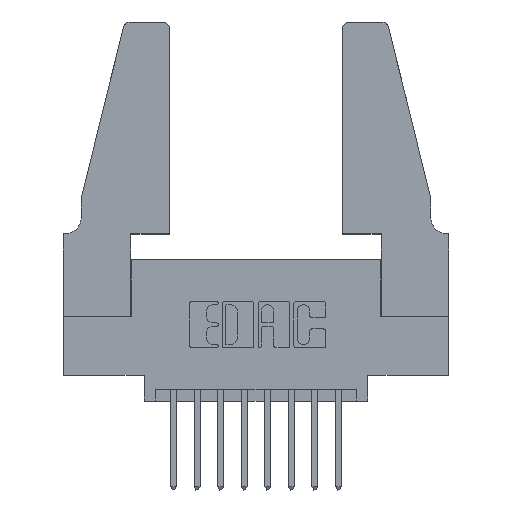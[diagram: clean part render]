
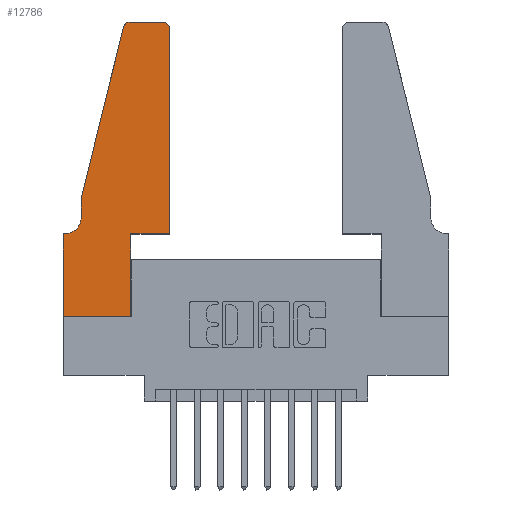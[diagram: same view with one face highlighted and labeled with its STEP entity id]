
A CAD part, top view. The second image highlights one B-rep face of the part: STEP entity #12786.
In plain terms, the highlighted planar face has unit normal (0, 0, 1).
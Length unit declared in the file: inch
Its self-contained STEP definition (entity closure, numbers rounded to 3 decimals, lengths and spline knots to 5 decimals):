
#7 = DIRECTION ( 'NONE',  ( 0., 1., 0. ) ) ;
#111 = CARTESIAN_POINT ( 'NONE',  ( 0.284, 1.22, 0.37 ) ) ;
#139 = VECTOR ( 'NONE', #7, 39.37008 ) ;
#411 = VERTEX_POINT ( 'NONE', #1098 ) ;
#494 = LINE ( 'NONE', #7327, #139 ) ;
#654 = ORIENTED_EDGE ( 'NONE', *, *, #11352, .T. ) ;
#858 = LINE ( 'NONE', #7515, #8776 ) ;
#988 = DIRECTION ( 'NONE',  ( -1., 0., 0. ) ) ;
#1098 = CARTESIAN_POINT ( 'NONE',  ( 0.284, 1.25, 0.37 ) ) ;
#1178 = VECTOR ( 'NONE', #6517, 39.37008 ) ;
#1212 = DIRECTION ( 'NONE',  ( 1., 0., 0. ) ) ;
#1305 = DIRECTION ( 'NONE',  ( 0., -1., 0. ) ) ;
#1390 = ORIENTED_EDGE ( 'NONE', *, *, #6746, .T. ) ;
#1464 = CARTESIAN_POINT ( 'NONE',  ( 0.4505, 0.35, 0.37 ) ) ;
#1557 = ORIENTED_EDGE ( 'NONE', *, *, #8602, .T. ) ;
#1567 = CARTESIAN_POINT ( 'NONE',  ( 0.0055, 0.42, 0.37 ) ) ;
#1568 = EDGE_LOOP ( 'NONE', ( #2621, #1390, #12652, #9946, #3167, #3670, #12107, #654, #2486, #9514, #1557, #12460 ) ) ;
#2068 = CARTESIAN_POINT ( 'NONE',  ( 0.0755, 0.35, 0.37 ) ) ;
#2070 = AXIS2_PLACEMENT_3D ( 'NONE', #9506, #10512, #4467 ) ;
#2393 = PLANE ( 'NONE',  #2070 ) ;
#2395 = LINE ( 'NONE', #2068, #12779 ) ;
#2486 = ORIENTED_EDGE ( 'NONE', *, *, #5365, .T. ) ;
#2611 = CARTESIAN_POINT ( 'NONE',  ( 0.2865, 0.35, 0.37 ) ) ;
#2621 = ORIENTED_EDGE ( 'NONE', *, *, #4824, .T. ) ;
#2660 = DIRECTION ( 'NONE',  ( -1., 0., 0. ) ) ;
#2668 = VECTOR ( 'NONE', #8223, 39.37008 ) ;
#3029 = LINE ( 'NONE', #4763, #10786 ) ;
#3167 = ORIENTED_EDGE ( 'NONE', *, *, #9103, .T. ) ;
#3335 = VECTOR ( 'NONE', #6585, 39.37008 ) ;
#3392 = VERTEX_POINT ( 'NONE', #5178 ) ;
#3670 = ORIENTED_EDGE ( 'NONE', *, *, #4068, .T. ) ;
#3869 = DIRECTION ( 'NONE',  ( 0., 0., 1. ) ) ;
#4068 = EDGE_CURVE ( 'NONE', #4286, #9847, #2395, .T. ) ;
#4286 = VERTEX_POINT ( 'NONE', #10531 ) ;
#4381 = AXIS2_PLACEMENT_3D ( 'NONE', #111, #7429, #1212 ) ;
#4429 = CARTESIAN_POINT ( 'NONE',  ( 0.2605, 1.25, 0.37 ) ) ;
#4467 = DIRECTION ( 'NONE',  ( 1., 0., 0. ) ) ;
#4750 = EDGE_CURVE ( 'NONE', #7225, #6259, #4949, .T. ) ;
#4763 = CARTESIAN_POINT ( 'NONE',  ( 0.4505, 0.35, 0.37 ) ) ;
#4824 = EDGE_CURVE ( 'NONE', #3392, #411, #9364, .T. ) ;
#4949 = LINE ( 'NONE', #12377, #9997 ) ;
#4995 = CARTESIAN_POINT ( 'NONE',  ( 0.0755, 0.42, 0.37 ) ) ;
#5055 = CARTESIAN_POINT ( 'NONE',  ( 0., 0., 0.37 ) ) ;
#5178 = CARTESIAN_POINT ( 'NONE',  ( 0.4205, 1.25, 0.37 ) ) ;
#5207 = LINE ( 'NONE', #7580, #12853 ) ;
#5365 = EDGE_CURVE ( 'NONE', #11943, #7225, #494, .T. ) ;
#5390 = LINE ( 'NONE', #13116, #2668 ) ;
#5442 = CARTESIAN_POINT ( 'NONE',  ( 0.25487, 1.22718, 0.37 ) ) ;
#5466 = VERTEX_POINT ( 'NONE', #10550 ) ;
#5660 = CARTESIAN_POINT ( 'NONE',  ( 0.2865, 0., 0.37 ) ) ;
#6254 = CARTESIAN_POINT ( 'NONE',  ( 0., 0.35, 0.37 ) ) ;
#6259 = VERTEX_POINT ( 'NONE', #1464 ) ;
#6517 = DIRECTION ( 'NONE',  ( -1., 0., 0. ) ) ;
#6585 = DIRECTION ( 'NONE',  ( 0., -1., 0. ) ) ;
#6746 = EDGE_CURVE ( 'NONE', #411, #11276, #12376, .T. ) ;
#7225 = VERTEX_POINT ( 'NONE', #2611 ) ;
#7327 = CARTESIAN_POINT ( 'NONE',  ( 0.2865, 0.35, 0.37 ) ) ;
#7429 = DIRECTION ( 'NONE',  ( 0., 0., 1. ) ) ;
#7432 = DIRECTION ( 'NONE',  ( 1., 0., 0. ) ) ;
#7454 = VERTEX_POINT ( 'NONE', #5055 ) ;
#7515 = CARTESIAN_POINT ( 'NONE',  ( 0., 0., 0.37 ) ) ;
#7580 = CARTESIAN_POINT ( 'NONE',  ( 0., 0., 0.37 ) ) ;
#7748 = EDGE_CURVE ( 'NONE', #9847, #7454, #858, .T. ) ;
#7817 = CIRCLE ( 'NONE', #12066, 0.07 ) ;
#8120 = VERTEX_POINT ( 'NONE', #4995 ) ;
#8223 = DIRECTION ( 'NONE',  ( -0.239, -0.971, 0. ) ) ;
#8602 = EDGE_CURVE ( 'NONE', #6259, #5466, #3029, .T. ) ;
#8738 = LINE ( 'NONE', #12514, #3335 ) ;
#8741 = DIRECTION ( 'NONE',  ( 0., 0., -1. ) ) ;
#8776 = VECTOR ( 'NONE', #1305, 39.37008 ) ;
#8791 = DIRECTION ( 'NONE',  ( 0., 1., 0. ) ) ;
#9001 = AXIS2_PLACEMENT_3D ( 'NONE', #9943, #3869, #10959 ) ;
#9026 = EDGE_CURVE ( 'NONE', #12823, #8120, #8738, .T. ) ;
#9103 = EDGE_CURVE ( 'NONE', #8120, #4286, #7817, .T. ) ;
#9364 = LINE ( 'NONE', #4429, #1178 ) ;
#9506 = CARTESIAN_POINT ( 'NONE',  ( 0., 0.35, 0.37 ) ) ;
#9514 = ORIENTED_EDGE ( 'NONE', *, *, #4750, .T. ) ;
#9590 = FACE_OUTER_BOUND ( 'NONE', #1568, .T. ) ;
#9764 = CIRCLE ( 'NONE', #9001, 0.03 ) ;
#9847 = VERTEX_POINT ( 'NONE', #6254 ) ;
#9943 = CARTESIAN_POINT ( 'NONE',  ( 0.4205, 1.22, 0.37 ) ) ;
#9946 = ORIENTED_EDGE ( 'NONE', *, *, #9026, .T. ) ;
#9997 = VECTOR ( 'NONE', #7432, 39.37008 ) ;
#10512 = DIRECTION ( 'NONE',  ( 0., 0., 1. ) ) ;
#10531 = CARTESIAN_POINT ( 'NONE',  ( 0.0055, 0.35, 0.37 ) ) ;
#10550 = CARTESIAN_POINT ( 'NONE',  ( 0.4505, 1.22, 0.37 ) ) ;
#10562 = CARTESIAN_POINT ( 'NONE',  ( 0.0755, 0.5, 0.37 ) ) ;
#10786 = VECTOR ( 'NONE', #8791, 39.37008 ) ;
#10959 = DIRECTION ( 'NONE',  ( 1., 0., 0. ) ) ;
#11124 = EDGE_CURVE ( 'NONE', #11276, #12823, #5390, .T. ) ;
#11276 = VERTEX_POINT ( 'NONE', #5442 ) ;
#11352 = EDGE_CURVE ( 'NONE', #7454, #11943, #5207, .T. ) ;
#11943 = VERTEX_POINT ( 'NONE', #5660 ) ;
#12066 = AXIS2_PLACEMENT_3D ( 'NONE', #1567, #8741, #2660 ) ;
#12090 = EDGE_CURVE ( 'NONE', #5466, #3392, #9764, .T. ) ;
#12107 = ORIENTED_EDGE ( 'NONE', *, *, #7748, .T. ) ;
#12376 = CIRCLE ( 'NONE', #4381, 0.03 ) ;
#12377 = CARTESIAN_POINT ( 'NONE',  ( 0.4505, 0.35, 0.37 ) ) ;
#12460 = ORIENTED_EDGE ( 'NONE', *, *, #12090, .T. ) ;
#12512 = DIRECTION ( 'NONE',  ( 1., 0., 0. ) ) ;
#12514 = CARTESIAN_POINT ( 'NONE',  ( 0.0755, 0.5, 0.37 ) ) ;
#12652 = ORIENTED_EDGE ( 'NONE', *, *, #11124, .T. ) ;
#12779 = VECTOR ( 'NONE', #988, 39.37008 ) ;
#12786 = ADVANCED_FACE ( 'NONE', ( #9590 ), #2393, .T. ) ;
#12823 = VERTEX_POINT ( 'NONE', #10562 ) ;
#12853 = VECTOR ( 'NONE', #12512, 39.37008 ) ;
#13116 = CARTESIAN_POINT ( 'NONE',  ( 0.0755, 0.5, 0.37 ) ) ;
